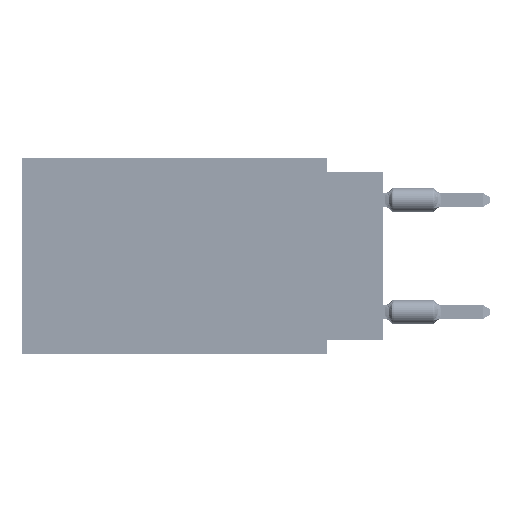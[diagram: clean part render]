
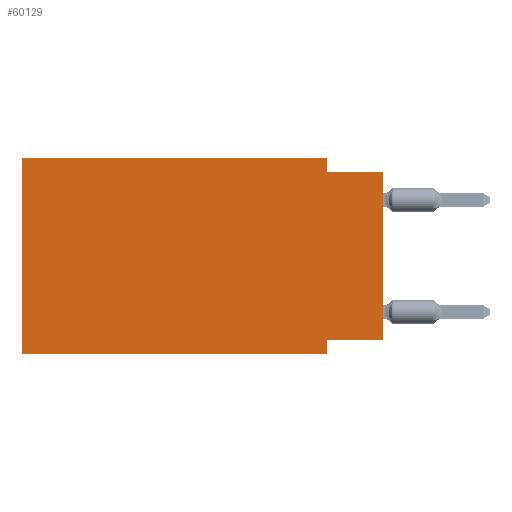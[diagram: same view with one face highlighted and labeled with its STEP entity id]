
A CAD part, left-side view. The second image highlights one B-rep face of the part: STEP entity #60129.
In plain terms, the highlighted planar face has unit normal (-1, 0, 0).
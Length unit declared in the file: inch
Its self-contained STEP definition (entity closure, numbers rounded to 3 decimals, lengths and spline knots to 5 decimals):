
#300 = EDGE_CURVE ( 'NONE', #33204, #61177, #90249, .T. ) ;
#1282 = CARTESIAN_POINT ( 'NONE',  ( 0., 0., -0.325 ) ) ;
#4032 = DIRECTION ( 'NONE',  ( 0., -1., 0. ) ) ;
#10513 = CARTESIAN_POINT ( 'NONE',  ( 0., 0.645, -0.35 ) ) ;
#12158 = VERTEX_POINT ( 'NONE', #1282 ) ;
#13824 = CARTESIAN_POINT ( 'NONE',  ( 0., 0.1, 0. ) ) ;
#15371 = ORIENTED_EDGE ( 'NONE', *, *, #72343, .F. ) ;
#16910 = ORIENTED_EDGE ( 'NONE', *, *, #95672, .F. ) ;
#17294 = LINE ( 'NONE', #26318, #67219 ) ;
#18614 = LINE ( 'NONE', #35529, #33679 ) ;
#19587 = DIRECTION ( 'NONE',  ( 1., 0., 0. ) ) ;
#20970 = DIRECTION ( 'NONE',  ( 0., 1., 0. ) ) ;
#23310 = EDGE_CURVE ( 'NONE', #12158, #26549, #17294, .T. ) ;
#23687 = LINE ( 'NONE', #83365, #59643 ) ;
#24129 = ORIENTED_EDGE ( 'NONE', *, *, #72107, .F. ) ;
#26199 = EDGE_CURVE ( 'NONE', #109873, #37611, #44215, .T. ) ;
#26318 = CARTESIAN_POINT ( 'NONE',  ( 0., 0., 0. ) ) ;
#26393 = DIRECTION ( 'NONE',  ( 0., 0., -1. ) ) ;
#26484 = CARTESIAN_POINT ( 'NONE',  ( 0., 0.1, -0.35 ) ) ;
#26549 = VERTEX_POINT ( 'NONE', #39997 ) ;
#26879 = VERTEX_POINT ( 'NONE', #55656 ) ;
#32950 = LINE ( 'NONE', #13824, #51835 ) ;
#33204 = VERTEX_POINT ( 'NONE', #10513 ) ;
#33464 = EDGE_CURVE ( 'NONE', #69136, #26879, #32950, .T. ) ;
#33679 = VECTOR ( 'NONE', #52965, 39.37008 ) ;
#35156 = ORIENTED_EDGE ( 'NONE', *, *, #26199, .F. ) ;
#35529 = CARTESIAN_POINT ( 'NONE',  ( 0., 0., -0.025 ) ) ;
#37611 = VERTEX_POINT ( 'NONE', #26484 ) ;
#39997 = CARTESIAN_POINT ( 'NONE',  ( 0., 0., -0.025 ) ) ;
#41393 = DIRECTION ( 'NONE',  ( 0., 0., -1. ) ) ;
#41457 = ORIENTED_EDGE ( 'NONE', *, *, #33464, .F. ) ;
#44215 = LINE ( 'NONE', #95415, #105445 ) ;
#47549 = VECTOR ( 'NONE', #4032, 39.37008 ) ;
#48477 = LINE ( 'NONE', #107028, #47549 ) ;
#49885 = AXIS2_PLACEMENT_3D ( 'NONE', #104038, #19587, #26393 ) ;
#51549 = DIRECTION ( 'NONE',  ( 0., 0., -1. ) ) ;
#51835 = VECTOR ( 'NONE', #41393, 39.37008 ) ;
#52965 = DIRECTION ( 'NONE',  ( 0., -1., 0. ) ) ;
#55656 = CARTESIAN_POINT ( 'NONE',  ( 0., 0.1, -0.025 ) ) ;
#59643 = VECTOR ( 'NONE', #82807, 39.37008 ) ;
#60129 = ADVANCED_FACE ( 'NONE', ( #78735 ), #97234, .F. ) ;
#61177 = VERTEX_POINT ( 'NONE', #98646 ) ;
#61201 = DIRECTION ( 'NONE',  ( 0., 0., 1. ) ) ;
#63767 = LINE ( 'NONE', #73877, #94728 ) ;
#64625 = ORIENTED_EDGE ( 'NONE', *, *, #300, .F. ) ;
#67219 = VECTOR ( 'NONE', #61201, 39.37008 ) ;
#69136 = VERTEX_POINT ( 'NONE', #94503 ) ;
#69738 = CARTESIAN_POINT ( 'NONE',  ( 0., 0.1, -0.325 ) ) ;
#72107 = EDGE_CURVE ( 'NONE', #12158, #109873, #63767, .T. ) ;
#72343 = EDGE_CURVE ( 'NONE', #26879, #26549, #18614, .T. ) ;
#73379 = DIRECTION ( 'NONE',  ( 0., 0., 1. ) ) ;
#73877 = CARTESIAN_POINT ( 'NONE',  ( 0., 0., -0.325 ) ) ;
#78735 = FACE_OUTER_BOUND ( 'NONE', #85239, .T. ) ;
#82807 = DIRECTION ( 'NONE',  ( 0., -1., 0. ) ) ;
#83365 = CARTESIAN_POINT ( 'NONE',  ( 0., 0.645, -0.35 ) ) ;
#85239 = EDGE_LOOP ( 'NONE', ( #109834, #15371, #41457, #16910, #64625, #109638, #35156, #24129 ) ) ;
#89707 = CARTESIAN_POINT ( 'NONE',  ( 0., 0.645, 0. ) ) ;
#90249 = LINE ( 'NONE', #89707, #95198 ) ;
#94503 = CARTESIAN_POINT ( 'NONE',  ( 0., 0.1, 0. ) ) ;
#94728 = VECTOR ( 'NONE', #20970, 39.37008 ) ;
#95198 = VECTOR ( 'NONE', #73379, 39.37008 ) ;
#95415 = CARTESIAN_POINT ( 'NONE',  ( 0., 0.1, -0.35 ) ) ;
#95672 = EDGE_CURVE ( 'NONE', #61177, #69136, #48477, .T. ) ;
#97234 = PLANE ( 'NONE',  #49885 ) ;
#98646 = CARTESIAN_POINT ( 'NONE',  ( 0., 0.645, 0. ) ) ;
#103285 = EDGE_CURVE ( 'NONE', #33204, #37611, #23687, .T. ) ;
#104038 = CARTESIAN_POINT ( 'NONE',  ( 0., 0.645, 0. ) ) ;
#105445 = VECTOR ( 'NONE', #51549, 39.37008 ) ;
#107028 = CARTESIAN_POINT ( 'NONE',  ( 0., 0.645, 0. ) ) ;
#109638 = ORIENTED_EDGE ( 'NONE', *, *, #103285, .T. ) ;
#109834 = ORIENTED_EDGE ( 'NONE', *, *, #23310, .T. ) ;
#109873 = VERTEX_POINT ( 'NONE', #69738 ) ;
